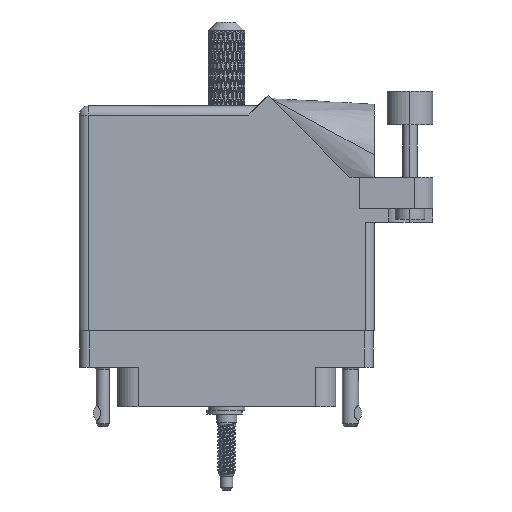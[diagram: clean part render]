
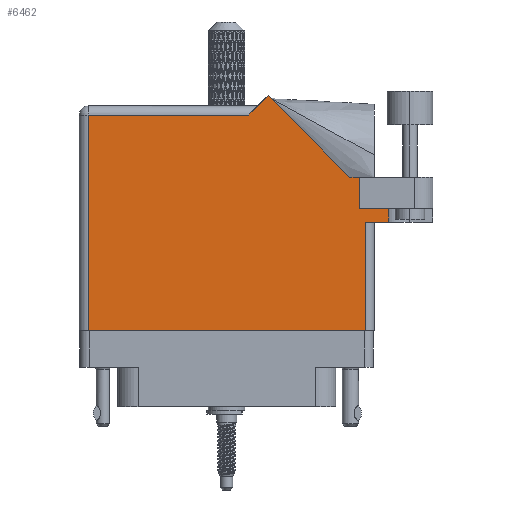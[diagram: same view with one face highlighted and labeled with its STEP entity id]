
A CAD part, front view. The second image highlights one B-rep face of the part: STEP entity #6462.
In plain terms, the highlighted face is planar.
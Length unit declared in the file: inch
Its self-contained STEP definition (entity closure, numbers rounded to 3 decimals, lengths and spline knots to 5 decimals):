
#1630 = EDGE_CURVE ( 'NONE', #20839, #4462, #82132, .T. ) ;
#1845 = DIRECTION ( 'NONE',  ( 1., 0., 0. ) ) ;
#3329 = AXIS2_PLACEMENT_3D ( 'NONE', #32223, #59846, #5643 ) ;
#4462 = VERTEX_POINT ( 'NONE', #111732 ) ;
#5643 = DIRECTION ( 'NONE',  ( -1., 0., 0. ) ) ;
#5904 = VECTOR ( 'NONE', #82101, 39.37008 ) ;
#6462 = ADVANCED_FACE ( 'NONE', ( #81307 ), #112319, .F. ) ;
#6733 = VERTEX_POINT ( 'NONE', #90882 ) ;
#7614 = ORIENTED_EDGE ( 'NONE', *, *, #75855, .T. ) ;
#7795 = DIRECTION ( 'NONE',  ( -0.707, -0.707, 0. ) ) ;
#8659 = LINE ( 'NONE', #107353, #15595 ) ;
#9018 = VERTEX_POINT ( 'NONE', #102841 ) ;
#9355 = ORIENTED_EDGE ( 'NONE', *, *, #1630, .F. ) ;
#15595 = VECTOR ( 'NONE', #1845, 39.37008 ) ;
#16186 = CARTESIAN_POINT ( 'NONE',  ( 0.905, 0.944, 0.455 ) ) ;
#16715 = CARTESIAN_POINT ( 'NONE',  ( 0.83942, 0.944, 0.455 ) ) ;
#17639 = EDGE_CURVE ( 'NONE', #109048, #50341, #84969, .T. ) ;
#19585 = CARTESIAN_POINT ( 'NONE',  ( 0.905, 0.731, 0.455 ) ) ;
#20839 = VERTEX_POINT ( 'NONE', #19585 ) ;
#21444 = LINE ( 'NONE', #47608, #82706 ) ;
#22235 = CARTESIAN_POINT ( 'NONE',  ( -1.005, 1.368, 0.455 ) ) ;
#22708 = LINE ( 'NONE', #45623, #5904 ) ;
#26120 = DIRECTION ( 'NONE',  ( 1., 0., 0. ) ) ;
#29040 = CARTESIAN_POINT ( 'NONE',  ( 1.1065, 1.06177, 0.455 ) ) ;
#29201 = ORIENTED_EDGE ( 'NONE', *, *, #104351, .T. ) ;
#31602 = DIRECTION ( 'NONE',  ( -1., 0., 0. ) ) ;
#32223 = CARTESIAN_POINT ( 'NONE',  ( -1.005, 1.43, 0.455 ) ) ;
#33685 = CARTESIAN_POINT ( 'NONE',  ( 0.905, 0.731, 0.455 ) ) ;
#34846 = VECTOR ( 'NONE', #97450, 39.37008 ) ;
#35157 = LINE ( 'NONE', #44808, #76875 ) ;
#38210 = CARTESIAN_POINT ( 'NONE',  ( 0.943, -0.1, 0.455 ) ) ;
#41936 = DIRECTION ( 'NONE',  ( -1., 0., 0. ) ) ;
#42546 = EDGE_CURVE ( 'NONE', #4462, #110441, #57719, .T. ) ;
#43287 = EDGE_CURVE ( 'NONE', #50341, #9018, #22708, .T. ) ;
#44687 = ORIENTED_EDGE ( 'NONE', *, *, #43287, .T. ) ;
#44808 = CARTESIAN_POINT ( 'NONE',  ( 0.212, 1.43, 0.455 ) ) ;
#45623 = CARTESIAN_POINT ( 'NONE',  ( 0.943, 0.637, 0.455 ) ) ;
#46587 = EDGE_CURVE ( 'NONE', #84533, #49560, #90502, .T. ) ;
#47608 = CARTESIAN_POINT ( 'NONE',  ( -0.943, -0.1, 0.455 ) ) ;
#47792 = EDGE_CURVE ( 'NONE', #6733, #84533, #35157, .T. ) ;
#47877 = ORIENTED_EDGE ( 'NONE', *, *, #46587, .T. ) ;
#49560 = VERTEX_POINT ( 'NONE', #76323 ) ;
#50341 = VERTEX_POINT ( 'NONE', #38210 ) ;
#51122 = VECTOR ( 'NONE', #41936, 39.37008 ) ;
#52941 = CARTESIAN_POINT ( 'NONE',  ( -0.943, -0.1, 0.455 ) ) ;
#54915 = ORIENTED_EDGE ( 'NONE', *, *, #71519, .T. ) ;
#56721 = LINE ( 'NONE', #33685, #84588 ) ;
#57719 = LINE ( 'NONE', #29040, #63246 ) ;
#58730 = CARTESIAN_POINT ( 'NONE',  ( 0.83942, 0.944, 0.455 ) ) ;
#59701 = ORIENTED_EDGE ( 'NONE', *, *, #42546, .F. ) ;
#59846 = DIRECTION ( 'NONE',  ( 0., 0., -1. ) ) ;
#60205 = EDGE_CURVE ( 'NONE', #108993, #6733, #83969, .T. ) ;
#60390 = CARTESIAN_POINT ( 'NONE',  ( -1.005, -0.1, 0.455 ) ) ;
#60807 = ORIENTED_EDGE ( 'NONE', *, *, #97151, .T. ) ;
#63246 = VECTOR ( 'NONE', #109188, 39.37008 ) ;
#67685 = DIRECTION ( 'NONE',  ( -0.707, 0.707, 0. ) ) ;
#67947 = EDGE_LOOP ( 'NONE', ( #103907, #44687, #29201, #59701, #9355, #54915, #60807, #84382, #110912, #47877, #7614 ) ) ;
#69283 = CARTESIAN_POINT ( 'NONE',  ( 0.15, 1.368, 0.455 ) ) ;
#71519 = EDGE_CURVE ( 'NONE', #20839, #97216, #56721, .T. ) ;
#75855 = EDGE_CURVE ( 'NONE', #49560, #109048, #21444, .T. ) ;
#76323 = CARTESIAN_POINT ( 'NONE',  ( -0.943, 1.368, 0.455 ) ) ;
#76875 = VECTOR ( 'NONE', #7795, 39.37008 ) ;
#81307 = FACE_OUTER_BOUND ( 'NONE', #67947, .T. ) ;
#81659 = CARTESIAN_POINT ( 'NONE',  ( 1.1065, 0.637, 0.455 ) ) ;
#82101 = DIRECTION ( 'NONE',  ( 0., 1., 0. ) ) ;
#82132 = LINE ( 'NONE', #85166, #34846 ) ;
#82706 = VECTOR ( 'NONE', #109795, 39.37008 ) ;
#83969 = LINE ( 'NONE', #58730, #114542 ) ;
#84382 = ORIENTED_EDGE ( 'NONE', *, *, #60205, .T. ) ;
#84533 = VERTEX_POINT ( 'NONE', #69283 ) ;
#84588 = VECTOR ( 'NONE', #85923, 39.37008 ) ;
#84969 = LINE ( 'NONE', #60390, #112734 ) ;
#85166 = CARTESIAN_POINT ( 'NONE',  ( 0.905, 0.731, 0.455 ) ) ;
#85923 = DIRECTION ( 'NONE',  ( 0., 1., 0. ) ) ;
#88738 = LINE ( 'NONE', #113042, #51122 ) ;
#90502 = LINE ( 'NONE', #22235, #108595 ) ;
#90882 = CARTESIAN_POINT ( 'NONE',  ( 0.28271, 1.50071, 0.455 ) ) ;
#97151 = EDGE_CURVE ( 'NONE', #97216, #108993, #88738, .T. ) ;
#97216 = VERTEX_POINT ( 'NONE', #16186 ) ;
#97450 = DIRECTION ( 'NONE',  ( 1., 0., 0. ) ) ;
#102841 = CARTESIAN_POINT ( 'NONE',  ( 0.943, 0.637, 0.455 ) ) ;
#103907 = ORIENTED_EDGE ( 'NONE', *, *, #17639, .T. ) ;
#104351 = EDGE_CURVE ( 'NONE', #9018, #110441, #8659, .T. ) ;
#107353 = CARTESIAN_POINT ( 'NONE',  ( 1.005, 0.637, 0.455 ) ) ;
#108595 = VECTOR ( 'NONE', #31602, 39.37008 ) ;
#108993 = VERTEX_POINT ( 'NONE', #16715 ) ;
#109048 = VERTEX_POINT ( 'NONE', #52941 ) ;
#109188 = DIRECTION ( 'NONE',  ( 0., -1., 0. ) ) ;
#109795 = DIRECTION ( 'NONE',  ( 0., -1., 0. ) ) ;
#110441 = VERTEX_POINT ( 'NONE', #81659 ) ;
#110912 = ORIENTED_EDGE ( 'NONE', *, *, #47792, .T. ) ;
#111732 = CARTESIAN_POINT ( 'NONE',  ( 1.1065, 0.731, 0.455 ) ) ;
#112319 = PLANE ( 'NONE',  #3329 ) ;
#112734 = VECTOR ( 'NONE', #26120, 39.37008 ) ;
#113042 = CARTESIAN_POINT ( 'NONE',  ( 1.405, 0.944, 0.455 ) ) ;
#114542 = VECTOR ( 'NONE', #67685, 39.37008 ) ;
